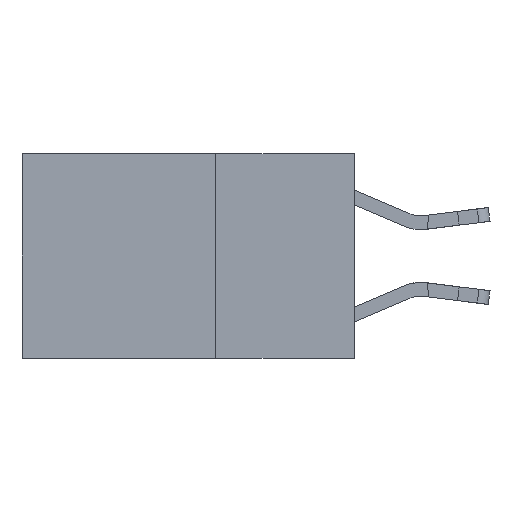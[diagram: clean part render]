
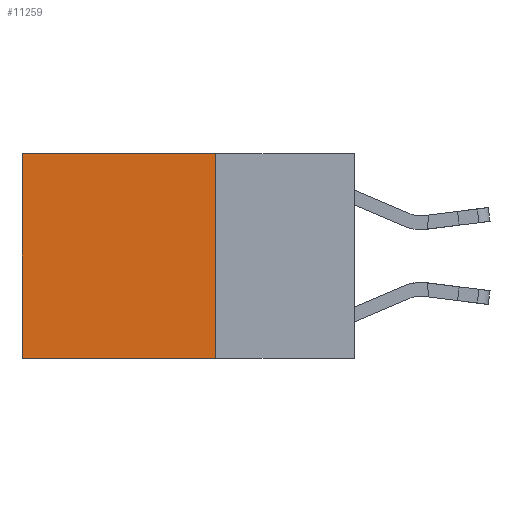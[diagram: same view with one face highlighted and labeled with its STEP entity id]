
A CAD part, left-side view. The second image highlights one B-rep face of the part: STEP entity #11259.
In plain terms, the highlighted planar face has unit normal (-1, 0, 0).
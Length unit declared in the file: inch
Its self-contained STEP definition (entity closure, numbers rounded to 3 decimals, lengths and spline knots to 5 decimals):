
#457 = DIRECTION ( 'NONE',  ( 1., 0., 0. ) ) ;
#853 = CARTESIAN_POINT ( 'NONE',  ( 0.2625, 0.6, 0. ) ) ;
#1907 = CARTESIAN_POINT ( 'NONE',  ( 0.2625, 0.25, 0. ) ) ;
#2919 = LINE ( 'NONE', #16102, #3086 ) ;
#3086 = VECTOR ( 'NONE', #6414, 39.37008 ) ;
#3906 = CARTESIAN_POINT ( 'NONE',  ( 0.2625, 0.6, 0. ) ) ;
#5953 = PLANE ( 'NONE',  #14348 ) ;
#6136 = VERTEX_POINT ( 'NONE', #7340 ) ;
#6192 = DIRECTION ( 'NONE',  ( 0., 0., -1. ) ) ;
#6414 = DIRECTION ( 'NONE',  ( 0., 0., -1. ) ) ;
#6422 = EDGE_LOOP ( 'NONE', ( #14969, #8914, #19106, #9415 ) ) ;
#6496 = CARTESIAN_POINT ( 'NONE',  ( 0.2625, 0.25, -0.37 ) ) ;
#7340 = CARTESIAN_POINT ( 'NONE',  ( 0.2625, 0.25, 0. ) ) ;
#7608 = FACE_OUTER_BOUND ( 'NONE', #6422, .T. ) ;
#8373 = DIRECTION ( 'NONE',  ( 0., 0., -1. ) ) ;
#8914 = ORIENTED_EDGE ( 'NONE', *, *, #18538, .F. ) ;
#9415 = ORIENTED_EDGE ( 'NONE', *, *, #16276, .T. ) ;
#11132 = VECTOR ( 'NONE', #8373, 39.37008 ) ;
#11259 = ADVANCED_FACE ( 'NONE', ( #7608 ), #5953, .F. ) ;
#12327 = EDGE_CURVE ( 'NONE', #16349, #16659, #22082, .T. ) ;
#12537 = LINE ( 'NONE', #6496, #16260 ) ;
#14305 = VERTEX_POINT ( 'NONE', #18390 ) ;
#14348 = AXIS2_PLACEMENT_3D ( 'NONE', #23443, #457, #6192 ) ;
#14969 = ORIENTED_EDGE ( 'NONE', *, *, #12327, .T. ) ;
#16005 = EDGE_CURVE ( 'NONE', #6136, #14305, #2919, .T. ) ;
#16102 = CARTESIAN_POINT ( 'NONE',  ( 0.2625, 0.25, 0. ) ) ;
#16260 = VECTOR ( 'NONE', #19671, 39.37008 ) ;
#16276 = EDGE_CURVE ( 'NONE', #6136, #16349, #19084, .T. ) ;
#16349 = VERTEX_POINT ( 'NONE', #3906 ) ;
#16659 = VERTEX_POINT ( 'NONE', #24617 ) ;
#17592 = DIRECTION ( 'NONE',  ( 0., 1., 0. ) ) ;
#18390 = CARTESIAN_POINT ( 'NONE',  ( 0.2625, 0.25, -0.37 ) ) ;
#18538 = EDGE_CURVE ( 'NONE', #14305, #16659, #12537, .T. ) ;
#19084 = LINE ( 'NONE', #1907, #22410 ) ;
#19106 = ORIENTED_EDGE ( 'NONE', *, *, #16005, .F. ) ;
#19671 = DIRECTION ( 'NONE',  ( 0., 1., 0. ) ) ;
#22082 = LINE ( 'NONE', #853, #11132 ) ;
#22410 = VECTOR ( 'NONE', #17592, 39.37008 ) ;
#23443 = CARTESIAN_POINT ( 'NONE',  ( 0.2625, 0.25, 0. ) ) ;
#24617 = CARTESIAN_POINT ( 'NONE',  ( 0.2625, 0.6, -0.37 ) ) ;
